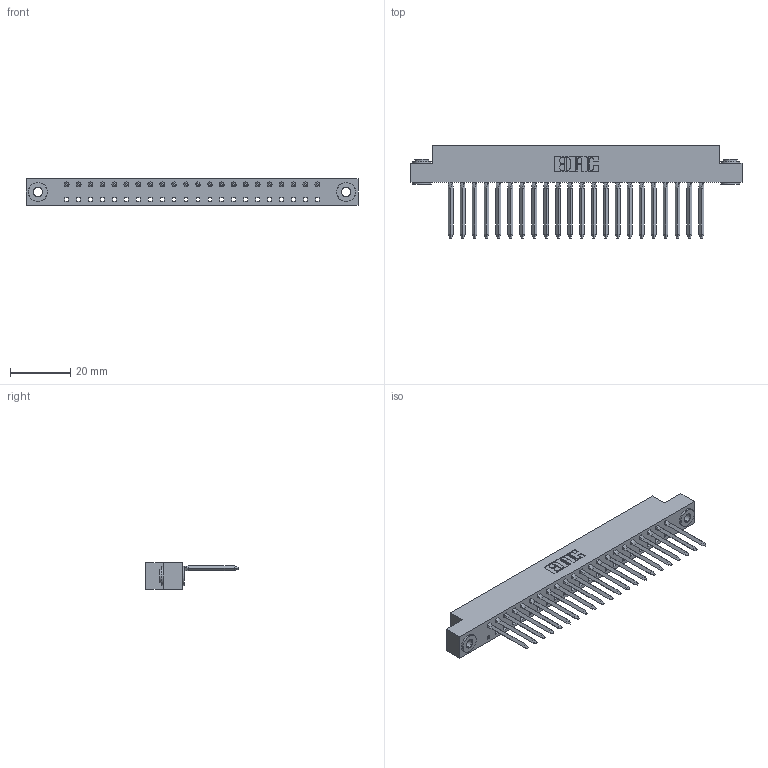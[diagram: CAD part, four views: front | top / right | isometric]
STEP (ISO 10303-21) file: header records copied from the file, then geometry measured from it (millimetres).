
FILE_DESCRIPTION (( 'STEP AP203' ), '1' );
FILE_NAME ('338-022-541-103.STEP', '2020-03-24T17:45:01', ( '' ), ( '' ), 'SwSTEP 2.0', 'SolidWorks 2016', '' );
FILE_SCHEMA (( 'CONFIG_CONTROL_DESIGN' ));
Length unit declared in the file: inch
Products named in the file (4): 345-250-002_345-250-002-102; 338-210-001_338-210-022-004; 338-290-001_541; 338-022-541-103
Assembly tree (25 placements, depth 2):
  338-022-541-103
    338-210-001_338-210-022-004
    338-290-001_541  x22
    345-250-002_345-250-002-102  x2
Bounding box: 110.19 x 30.56 x 8.71 mm (x, y, z)
Volume: 7713.8 mm3; surface area: 12672 mm2
Topology: 25 solids, 25 shells, 2192 faces, 6017 edges, 3846 vertices
Faces by surface type: plane 1504, cylinder 592, bspline 88, cone 8
Entity records: 45341 total; most frequent: CARTESIAN_POINT 9079, ORIENTED_EDGE 7632, DIRECTION 7141, EDGE_CURVE 3816, LINE 2829, VECTOR 2829, VERTEX_POINT 2478, AXIS2_PLACEMENT_3D 2156
